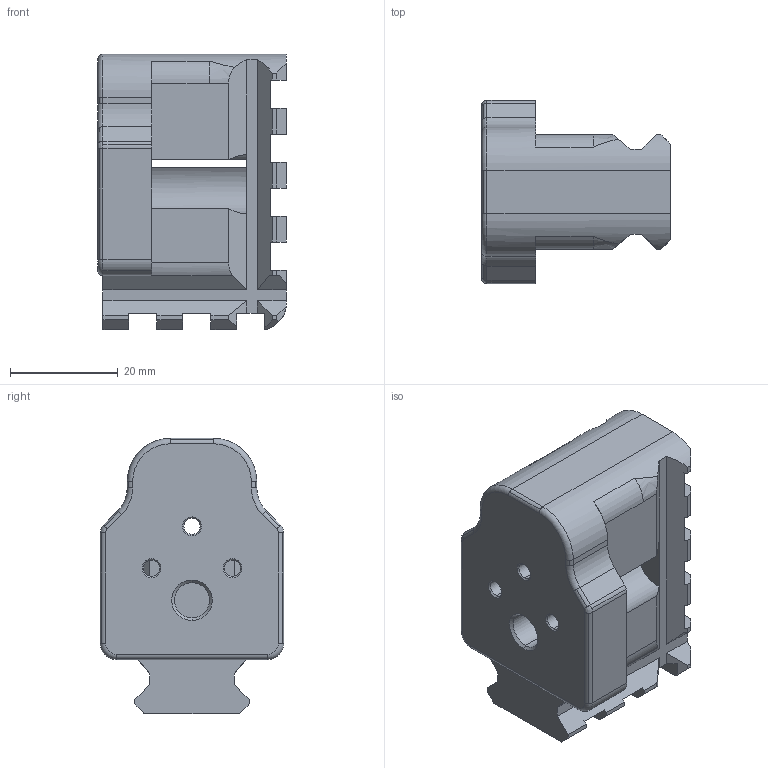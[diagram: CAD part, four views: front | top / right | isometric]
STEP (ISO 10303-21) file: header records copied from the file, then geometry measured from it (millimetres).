
FILE_DESCRIPTION (( 'STEP AP203' ), '1' );
FILE_NAME ('Brace_Adapter_1913.STEP', '2020-02-07T01:26:59', ( '' ), ( '' ), 'SwSTEP 2.0', 'SolidWorks 2019', '' );
FILE_SCHEMA (( 'CONFIG_CONTROL_DESIGN' ));
Length unit declared in the file: millimetre
Products named in the file (1): Brace_Adapter_1913
Bounding box: 35 x 34 x 51 mm (x, y, z)
Volume: 28833.5 mm3; surface area: 10990.6 mm2
Topology: 1 solids, 1 shells, 219 faces, 603 edges, 383 vertices
Faces by surface type: plane 116, cylinder 56, cone 22, bspline 13, torus 12
Entity records: 7275 total; most frequent: CARTESIAN_POINT 1654, ORIENTED_EDGE 1206, DIRECTION 1124, EDGE_CURVE 603, VERTEX_POINT 383, VECTOR 382, LINE 382, AXIS2_PLACEMENT_3D 371
